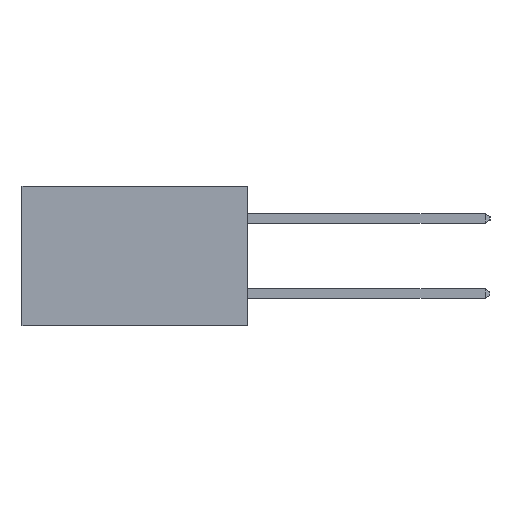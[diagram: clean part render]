
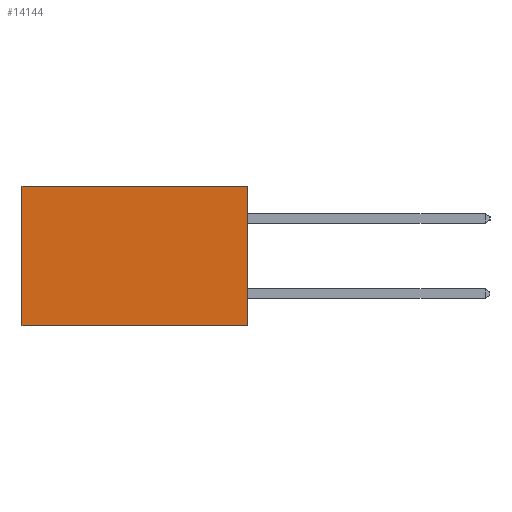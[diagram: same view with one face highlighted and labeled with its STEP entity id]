
A CAD part, left-side view. The second image highlights one B-rep face of the part: STEP entity #14144.
In plain terms, the highlighted planar face has unit normal (-1, 0, 0).
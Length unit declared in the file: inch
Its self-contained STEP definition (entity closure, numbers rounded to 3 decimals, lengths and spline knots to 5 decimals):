
#1415 = VERTEX_POINT ( 'NONE', #9516 ) ;
#1665 = DIRECTION ( 'NONE',  ( 0., 0., -1. ) ) ;
#1688 = DIRECTION ( 'NONE',  ( 0., 1., 0. ) ) ;
#2305 = VECTOR ( 'NONE', #1688, 39.37008 ) ;
#2682 = EDGE_CURVE ( 'NONE', #11776, #8479, #6234, .T. ) ;
#2958 = LINE ( 'NONE', #12023, #2305 ) ;
#3162 = EDGE_CURVE ( 'NONE', #1415, #23017, #21628, .T. ) ;
#3931 = ORIENTED_EDGE ( 'NONE', *, *, #2682, .F. ) ;
#4101 = FACE_OUTER_BOUND ( 'NONE', #16433, .T. ) ;
#4650 = EDGE_CURVE ( 'NONE', #8479, #23017, #20049, .T. ) ;
#6208 = VECTOR ( 'NONE', #19131, 39.37008 ) ;
#6234 = LINE ( 'NONE', #9626, #11673 ) ;
#6825 = ORIENTED_EDGE ( 'NONE', *, *, #4650, .F. ) ;
#8311 = CARTESIAN_POINT ( 'NONE',  ( 0.2615, 0., -0.37 ) ) ;
#8479 = VERTEX_POINT ( 'NONE', #8311 ) ;
#9086 = DIRECTION ( 'NONE',  ( 0., 1., 0. ) ) ;
#9236 = CARTESIAN_POINT ( 'NONE',  ( 0.2615, 0., -0.37 ) ) ;
#9367 = DIRECTION ( 'NONE',  ( 0., 0., -1. ) ) ;
#9516 = CARTESIAN_POINT ( 'NONE',  ( 0.2615, 0.6, 0. ) ) ;
#9626 = CARTESIAN_POINT ( 'NONE',  ( 0.2615, 0., -0.37 ) ) ;
#11673 = VECTOR ( 'NONE', #9367, 39.37008 ) ;
#11776 = VERTEX_POINT ( 'NONE', #15054 ) ;
#12023 = CARTESIAN_POINT ( 'NONE',  ( 0.2615, 0., 0. ) ) ;
#13994 = DIRECTION ( 'NONE',  ( 1., 0., 0. ) ) ;
#14144 = ADVANCED_FACE ( 'NONE', ( #4101 ), #25912, .F. ) ;
#15054 = CARTESIAN_POINT ( 'NONE',  ( 0.2615, 0., 0. ) ) ;
#15579 = ORIENTED_EDGE ( 'NONE', *, *, #17282, .T. ) ;
#16433 = EDGE_LOOP ( 'NONE', ( #22402, #6825, #3931, #15579 ) ) ;
#17282 = EDGE_CURVE ( 'NONE', #11776, #1415, #2958, .T. ) ;
#18272 = CARTESIAN_POINT ( 'NONE',  ( 0.2615, 0.6, -0.37 ) ) ;
#19131 = DIRECTION ( 'NONE',  ( 0., 0., -1. ) ) ;
#20049 = LINE ( 'NONE', #9236, #24681 ) ;
#20839 = CARTESIAN_POINT ( 'NONE',  ( 0.2615, 0.6, -0.37 ) ) ;
#21628 = LINE ( 'NONE', #18272, #6208 ) ;
#22402 = ORIENTED_EDGE ( 'NONE', *, *, #3162, .T. ) ;
#23017 = VERTEX_POINT ( 'NONE', #20839 ) ;
#24333 = AXIS2_PLACEMENT_3D ( 'NONE', #25826, #13994, #1665 ) ;
#24681 = VECTOR ( 'NONE', #9086, 39.37008 ) ;
#25826 = CARTESIAN_POINT ( 'NONE',  ( 0.2615, 0., -0.37 ) ) ;
#25912 = PLANE ( 'NONE',  #24333 ) ;
